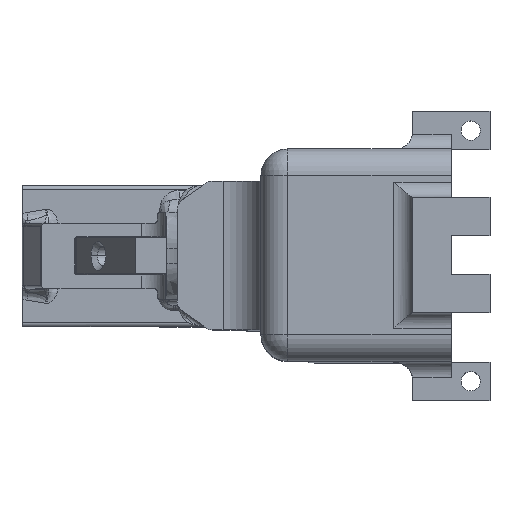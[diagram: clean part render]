
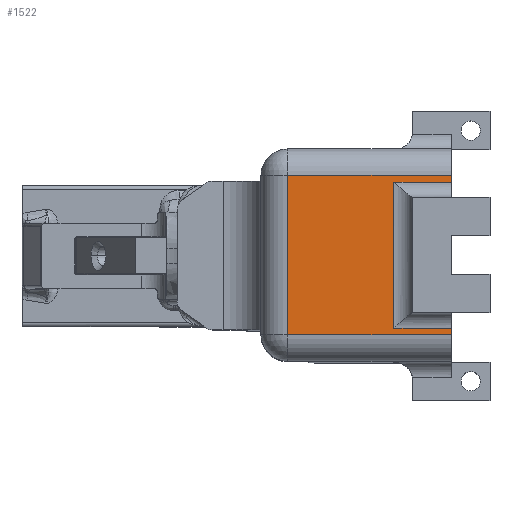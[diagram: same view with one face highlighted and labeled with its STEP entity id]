
A CAD part, top view. The second image highlights one B-rep face of the part: STEP entity #1522.
In plain terms, the highlighted planar face has unit normal (0, 0, 1).
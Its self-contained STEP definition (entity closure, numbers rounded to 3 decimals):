
#247 = DIRECTION ( 'NONE',  ( 0., 1., 0. ) ) ;
#908 = EDGE_CURVE ( 'NONE', #10940, #5109, #8897, .T. ) ;
#1028 = LINE ( 'NONE', #6845, #6396 ) ;
#1095 = ORIENTED_EDGE ( 'NONE', *, *, #10051, .T. ) ;
#1522 = ADVANCED_FACE ( 'NONE', ( #2135 ), #2969, .F. ) ;
#1575 = ORIENTED_EDGE ( 'NONE', *, *, #1634, .T. ) ;
#1634 = EDGE_CURVE ( 'NONE', #11477, #10940, #6749, .T. ) ;
#1768 = VERTEX_POINT ( 'NONE', #4538 ) ;
#2019 = CARTESIAN_POINT ( 'NONE',  ( 116.522, -20.148, 147.352 ) ) ;
#2086 = VECTOR ( 'NONE', #5581, 1000. ) ;
#2135 = FACE_OUTER_BOUND ( 'NONE', #4033, .T. ) ;
#2496 = ORIENTED_EDGE ( 'NONE', *, *, #5622, .T. ) ;
#2969 = PLANE ( 'NONE',  #7759 ) ;
#3076 = DIRECTION ( 'NONE',  ( 0., -1., 0. ) ) ;
#3230 = CARTESIAN_POINT ( 'NONE',  ( 73.323, 0., 147.352 ) ) ;
#3486 = EDGE_CURVE ( 'NONE', #14453, #9275, #14205, .T. ) ;
#4033 = EDGE_LOOP ( 'NONE', ( #10525, #1095, #8780, #15116, #7700, #1575, #14383, #2496 ) ) ;
#4072 = EDGE_CURVE ( 'NONE', #5759, #14453, #5348, .T. ) ;
#4189 = DIRECTION ( 'NONE',  ( 0., 0., -1. ) ) ;
#4538 = CARTESIAN_POINT ( 'NONE',  ( 116.522, -58.628, 147.352 ) ) ;
#4886 = CARTESIAN_POINT ( 'NONE',  ( 73.323, -60.353, 147.352 ) ) ;
#4894 = LINE ( 'NONE', #8531, #11650 ) ;
#4903 = DIRECTION ( 'NONE',  ( -1., 0., 0. ) ) ;
#5109 = VERTEX_POINT ( 'NONE', #9825 ) ;
#5286 = LINE ( 'NONE', #14942, #12416 ) ;
#5348 = LINE ( 'NONE', #7971, #2086 ) ;
#5540 = CARTESIAN_POINT ( 'NONE',  ( 101.362, -20.148, 147.352 ) ) ;
#5581 = DIRECTION ( 'NONE',  ( 1., 0., 0. ) ) ;
#5606 = VECTOR ( 'NONE', #11809, 1000. ) ;
#5622 = EDGE_CURVE ( 'NONE', #5109, #1768, #9630, .T. ) ;
#5759 = VERTEX_POINT ( 'NONE', #5540 ) ;
#5853 = DIRECTION ( 'NONE',  ( 0., 1., 0. ) ) ;
#5982 = DIRECTION ( 'NONE',  ( -1., 0., 0. ) ) ;
#6396 = VECTOR ( 'NONE', #5853, 1000. ) ;
#6661 = VECTOR ( 'NONE', #11137, 1000. ) ;
#6749 = LINE ( 'NONE', #3230, #15000 ) ;
#6845 = CARTESIAN_POINT ( 'NONE',  ( 101.362, -20.148, 147.352 ) ) ;
#7474 = EDGE_CURVE ( 'NONE', #1768, #13576, #4894, .T. ) ;
#7510 = EDGE_CURVE ( 'NONE', #9275, #11477, #5286, .T. ) ;
#7700 = ORIENTED_EDGE ( 'NONE', *, *, #7510, .T. ) ;
#7759 = AXIS2_PLACEMENT_3D ( 'NONE', #11551, #4189, #11652 ) ;
#7971 = CARTESIAN_POINT ( 'NONE',  ( 0., -20.148, 147.352 ) ) ;
#8531 = CARTESIAN_POINT ( 'NONE',  ( 106.362, -58.628, 147.352 ) ) ;
#8780 = ORIENTED_EDGE ( 'NONE', *, *, #4072, .T. ) ;
#8897 = LINE ( 'NONE', #10564, #5606 ) ;
#9121 = CARTESIAN_POINT ( 'NONE',  ( 73.323, -18.424, 147.352 ) ) ;
#9275 = VERTEX_POINT ( 'NONE', #15242 ) ;
#9630 = LINE ( 'NONE', #12415, #6661 ) ;
#9825 = CARTESIAN_POINT ( 'NONE',  ( 116.522, -60.353, 147.352 ) ) ;
#10051 = EDGE_CURVE ( 'NONE', #13576, #5759, #1028, .T. ) ;
#10525 = ORIENTED_EDGE ( 'NONE', *, *, #7474, .T. ) ;
#10564 = CARTESIAN_POINT ( 'NONE',  ( 116.522, -60.353, 147.352 ) ) ;
#10937 = CARTESIAN_POINT ( 'NONE',  ( 101.362, -58.628, 147.352 ) ) ;
#10940 = VERTEX_POINT ( 'NONE', #4886 ) ;
#11137 = DIRECTION ( 'NONE',  ( 0., 1., 0. ) ) ;
#11477 = VERTEX_POINT ( 'NONE', #9121 ) ;
#11551 = CARTESIAN_POINT ( 'NONE',  ( 0., 0., 147.352 ) ) ;
#11650 = VECTOR ( 'NONE', #5982, 1000. ) ;
#11652 = DIRECTION ( 'NONE',  ( -1., 0., 0. ) ) ;
#11809 = DIRECTION ( 'NONE',  ( 1., 0., 0. ) ) ;
#12415 = CARTESIAN_POINT ( 'NONE',  ( 116.522, -11.424, 147.352 ) ) ;
#12416 = VECTOR ( 'NONE', #4903, 1000. ) ;
#13576 = VERTEX_POINT ( 'NONE', #10937 ) ;
#13710 = CARTESIAN_POINT ( 'NONE',  ( 116.522, -11.424, 147.352 ) ) ;
#14205 = LINE ( 'NONE', #13710, #14386 ) ;
#14383 = ORIENTED_EDGE ( 'NONE', *, *, #908, .T. ) ;
#14386 = VECTOR ( 'NONE', #247, 1000. ) ;
#14453 = VERTEX_POINT ( 'NONE', #2019 ) ;
#14942 = CARTESIAN_POINT ( 'NONE',  ( 73.323, -18.424, 147.352 ) ) ;
#15000 = VECTOR ( 'NONE', #3076, 1000. ) ;
#15116 = ORIENTED_EDGE ( 'NONE', *, *, #3486, .T. ) ;
#15242 = CARTESIAN_POINT ( 'NONE',  ( 116.522, -18.424, 147.352 ) ) ;
